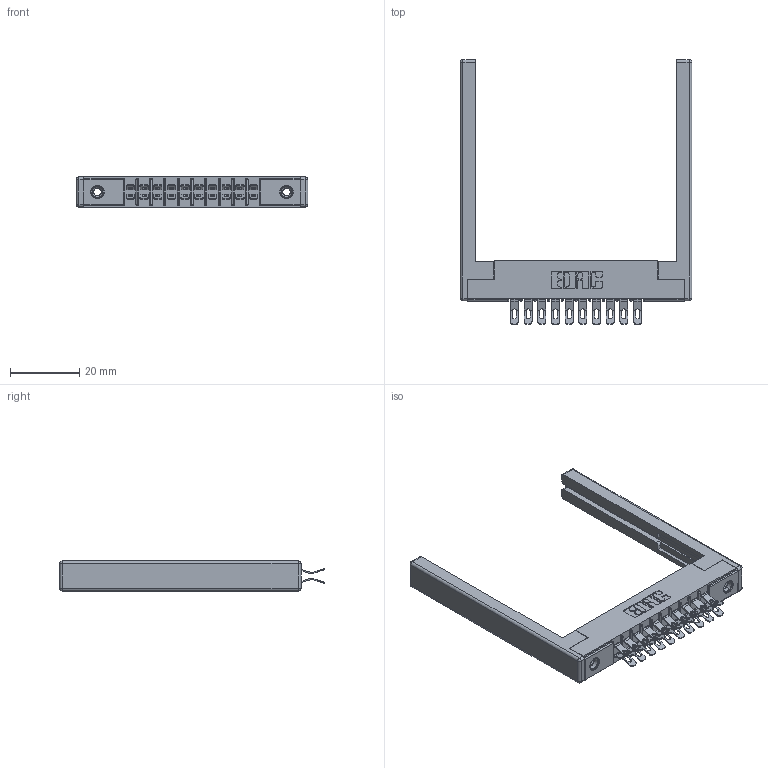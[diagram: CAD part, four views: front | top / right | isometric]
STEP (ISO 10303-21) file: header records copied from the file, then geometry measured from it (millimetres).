
FILE_DESCRIPTION (( 'STEP AP203' ), '1' );
FILE_NAME ('315-020-555-268.STEP', '2019-09-10T14:17:31', ( '' ), ( '' ), 'SwSTEP 2.0', 'SolidWorks 2016', '' );
FILE_SCHEMA (( 'CONFIG_CONTROL_DESIGN' ));
Length unit declared in the file: inch
Products named in the file (5): 315-020-555-268; 345-250-001_345-250-001-102; 305-290-001_555; 307-220-068; 305 Part_.156 Dia
Assembly tree (25 placements, depth 2):
  315-020-555-268
    305 Part_.156 Dia
    305-290-001_555  x20
    345-250-001_345-250-001-102  x2
    307-220-068  x2
Bounding box: 67.06 x 76.71 x 8.71 mm (x, y, z)
Volume: 8860.3 mm3; surface area: 11749 mm2
Topology: 25 solids, 25 shells, 1590 faces, 4656 edges, 3028 vertices
Faces by surface type: plane 796, cylinder 730, sphere 48, cone 12, torus 4
Entity records: 18106 total; most frequent: CARTESIAN_POINT 2987, ORIENTED_EDGE 2942, DIRECTION 2929, EDGE_CURVE 1471, VECTOR 1125, LINE 1125, VERTEX_POINT 944, AXIS2_PLACEMENT_3D 902
